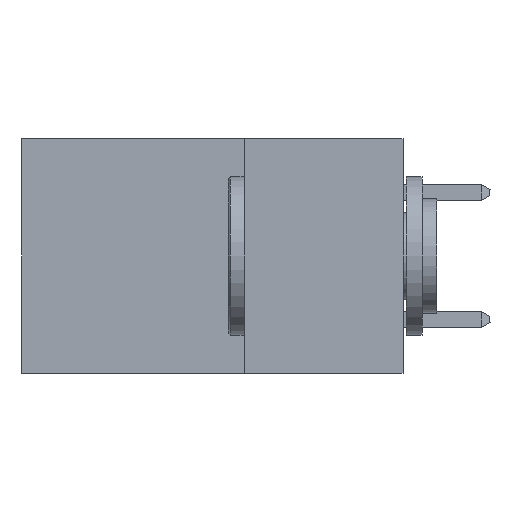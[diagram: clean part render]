
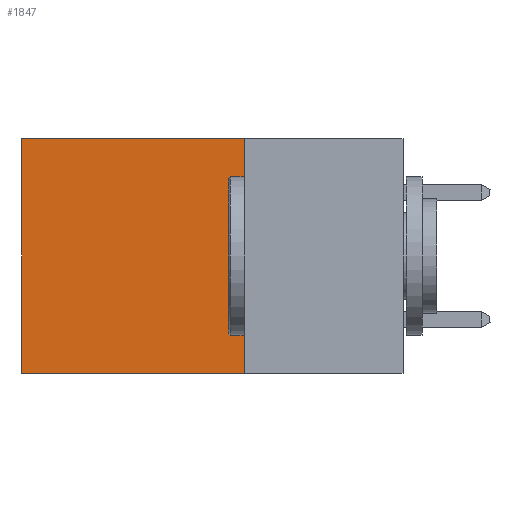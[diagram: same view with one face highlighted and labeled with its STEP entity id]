
A CAD part, left-side view. The second image highlights one B-rep face of the part: STEP entity #1847.
In plain terms, the highlighted planar face has unit normal (-1, 0, 0).
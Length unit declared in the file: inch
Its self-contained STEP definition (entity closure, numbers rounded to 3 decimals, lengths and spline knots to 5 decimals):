
#346 = CARTESIAN_POINT ( 'NONE',  ( 0.2875, 0.25, 0. ) ) ;
#622 = CARTESIAN_POINT ( 'NONE',  ( 0.2875, 0.25, 0. ) ) ;
#1847 = ADVANCED_FACE ( 'NONE', ( #8074 ), #2656, .F. ) ;
#2040 = ORIENTED_EDGE ( 'NONE', *, *, #5124, .T. ) ;
#2341 = EDGE_CURVE ( 'NONE', #8967, #7354, #7388, .T. ) ;
#2589 = ORIENTED_EDGE ( 'NONE', *, *, #2341, .T. ) ;
#2633 = CARTESIAN_POINT ( 'NONE',  ( 0.2875, 0.6, 0. ) ) ;
#2637 = DIRECTION ( 'NONE',  ( 0., 1., 0. ) ) ;
#2656 = PLANE ( 'NONE',  #13680 ) ;
#2722 = CARTESIAN_POINT ( 'NONE',  ( 0.2875, 0.25, -0.37 ) ) ;
#3320 = CARTESIAN_POINT ( 'NONE',  ( 0.2875, 0.6, -0.37 ) ) ;
#3398 = VECTOR ( 'NONE', #7030, 39.37008 ) ;
#3493 = LINE ( 'NONE', #622, #14085 ) ;
#3722 = DIRECTION ( 'NONE',  ( 0., 0., -1. ) ) ;
#3745 = DIRECTION ( 'NONE',  ( 0., 0., -1. ) ) ;
#3921 = ORIENTED_EDGE ( 'NONE', *, *, #5060, .F. ) ;
#4867 = EDGE_CURVE ( 'NONE', #10112, #11633, #5623, .T. ) ;
#4975 = CARTESIAN_POINT ( 'NONE',  ( 0.2875, 0.25, -0.37 ) ) ;
#5060 = EDGE_CURVE ( 'NONE', #8967, #10112, #3493, .T. ) ;
#5124 = EDGE_CURVE ( 'NONE', #7354, #11633, #13809, .T. ) ;
#5623 = LINE ( 'NONE', #2722, #8163 ) ;
#5866 = CARTESIAN_POINT ( 'NONE',  ( 0.2875, 0.25, 0. ) ) ;
#5907 = DIRECTION ( 'NONE',  ( 1., 0., 0. ) ) ;
#7030 = DIRECTION ( 'NONE',  ( 0., 0., -1. ) ) ;
#7354 = VERTEX_POINT ( 'NONE', #7678 ) ;
#7388 = LINE ( 'NONE', #11479, #9763 ) ;
#7678 = CARTESIAN_POINT ( 'NONE',  ( 0.2875, 0.6, 0. ) ) ;
#8074 = FACE_OUTER_BOUND ( 'NONE', #12026, .T. ) ;
#8163 = VECTOR ( 'NONE', #2637, 39.37008 ) ;
#8626 = ORIENTED_EDGE ( 'NONE', *, *, #4867, .F. ) ;
#8967 = VERTEX_POINT ( 'NONE', #346 ) ;
#9763 = VECTOR ( 'NONE', #10412, 39.37008 ) ;
#10112 = VERTEX_POINT ( 'NONE', #4975 ) ;
#10412 = DIRECTION ( 'NONE',  ( 0., 1., 0. ) ) ;
#11479 = CARTESIAN_POINT ( 'NONE',  ( 0.2875, 0.25, 0. ) ) ;
#11633 = VERTEX_POINT ( 'NONE', #3320 ) ;
#12026 = EDGE_LOOP ( 'NONE', ( #2040, #8626, #3921, #2589 ) ) ;
#13680 = AXIS2_PLACEMENT_3D ( 'NONE', #5866, #5907, #3745 ) ;
#13809 = LINE ( 'NONE', #2633, #3398 ) ;
#14085 = VECTOR ( 'NONE', #3722, 39.37008 ) ;
